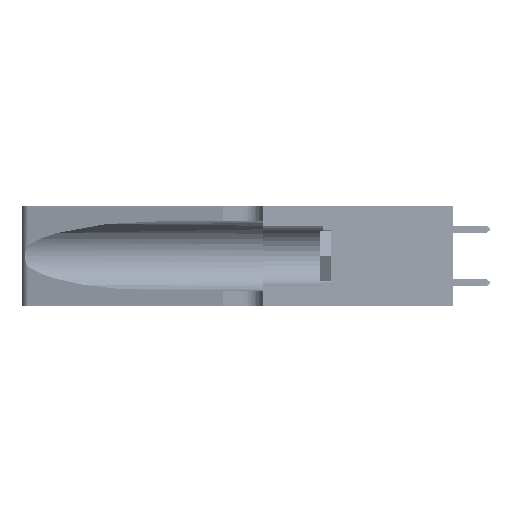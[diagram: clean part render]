
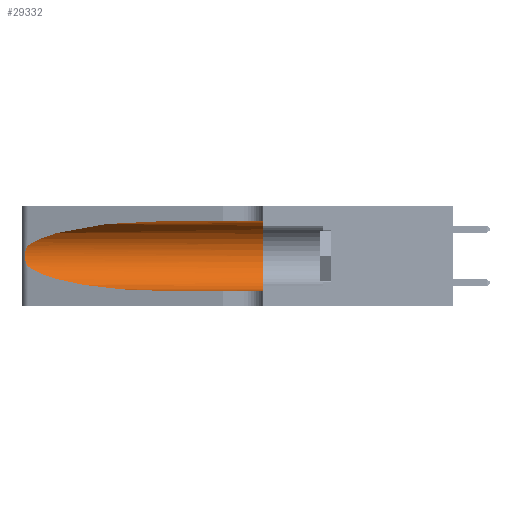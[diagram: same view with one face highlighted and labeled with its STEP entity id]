
A CAD part, left-side view. The second image highlights one B-rep face of the part: STEP entity #29332.
In plain terms, the highlighted cylindrical face has radius 3.308 mm (diameter 6.617 mm), a partial arc.
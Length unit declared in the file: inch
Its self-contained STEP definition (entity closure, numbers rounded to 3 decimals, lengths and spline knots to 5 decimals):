
#169 = CARTESIAN_POINT ( 'NONE',  ( 0.1305, 0.35, 0.31525 ) ) ;
#1890 = VERTEX_POINT ( 'NONE', #169 ) ;
#1937 = CARTESIAN_POINT ( 'NONE',  ( 0.25555, 1.22993, 0.14849 ) ) ;
#3401 = VECTOR ( 'NONE', #18199, 39.37008 ) ;
#4454 = CARTESIAN_POINT ( 'NONE',  ( 0.1305, 0.35, 0.185 ) ) ;
#5947 = CARTESIAN_POINT ( 'NONE',  ( 0.25555, 1.22994, 0.2215 ) ) ;
#6006 = VERTEX_POINT ( 'NONE', #49489 ) ;
#6018 = LINE ( 'NONE', #13987, #3401 ) ;
#6129 = EDGE_CURVE ( 'NONE', #32163, #25042, #22396, .T. ) ;
#7851 =( BOUNDED_CURVE ( )  B_SPLINE_CURVE ( 3, ( #29032, #51303, #33178, #8228 ),
 .UNSPECIFIED., .F., .T. ) 
 B_SPLINE_CURVE_WITH_KNOTS ( ( 4, 4 ),
 ( 1.5708, 2.84003 ),
 .UNSPECIFIED. ) 
 CURVE ( )  GEOMETRIC_REPRESENTATION_ITEM ( )  RATIONAL_B_SPLINE_CURVE ( ( 1., 0.87, 0.87, 1. ) ) 
 REPRESENTATION_ITEM ( '' )  );
#8228 = CARTESIAN_POINT ( 'NONE',  ( 0.25487, 1.22718, 0.22369 ) ) ;
#8542 = LINE ( 'NONE', #27172, #42915 ) ;
#8654 = DIRECTION ( 'NONE',  ( 0., 0., 1. ) ) ;
#10156 = CARTESIAN_POINT ( 'NONE',  ( 0.25787, 1.23484, 0.2124 ) ) ;
#10996 = ORIENTED_EDGE ( 'NONE', *, *, #44188, .F. ) ;
#11939 = CYLINDRICAL_SURFACE ( 'NONE', #45114, 0.13025 ) ;
#12152 = CARTESIAN_POINT ( 'NONE',  ( 0.25487, 1.22718, 0.22369 ) ) ;
#12495 = EDGE_CURVE ( 'NONE', #1890, #6006, #49805, .T. ) ;
#12565 = CARTESIAN_POINT ( 'NONE',  ( 0.1305, 0.72297, 0.31525 ) ) ;
#12991 = CARTESIAN_POINT ( 'NONE',  ( 0.18966, 0.96281, 0.05475 ) ) ;
#13987 = CARTESIAN_POINT ( 'NONE',  ( 0.1305, 1.61858, 0.05475 ) ) ;
#14342 = CARTESIAN_POINT ( 'NONE',  ( 0.26018, 1.23835, 0.19895 ) ) ;
#16954 = VERTEX_POINT ( 'NONE', #12565 ) ;
#17201 = CARTESIAN_POINT ( 'NONE',  ( 0.1305, 0.72297, 0.05475 ) ) ;
#18199 = DIRECTION ( 'NONE',  ( 0., -1., 0. ) ) ;
#18373 = CARTESIAN_POINT ( 'NONE',  ( 0.1305, 1.61858, 0.185 ) ) ;
#18577 = CARTESIAN_POINT ( 'NONE',  ( 0.26075, 1.23896, 0.178 ) ) ;
#22396 =( BOUNDED_CURVE ( )  B_SPLINE_CURVE ( 3, ( #41966, #37869, #12991, #17201 ),
 .UNSPECIFIED., .F., .F. ) 
 B_SPLINE_CURVE_WITH_KNOTS ( ( 4, 4 ),
 ( 3.44316, 4.71239 ),
 .UNSPECIFIED. ) 
 CURVE ( )  GEOMETRIC_REPRESENTATION_ITEM ( )  RATIONAL_B_SPLINE_CURVE ( ( 1., 0.87, 0.87, 1. ) ) 
 REPRESENTATION_ITEM ( '' )  );
#22766 = CARTESIAN_POINT ( 'NONE',  ( 0.25856, 1.23593, 0.16098 ) ) ;
#25042 = VERTEX_POINT ( 'NONE', #27680 ) ;
#25709 = B_SPLINE_CURVE_WITH_KNOTS ( 'NONE', 3,
 ( #30959, #5947, #35097, #10156, #39177, #14342, #43284, #18577, #47398, #22766, #51499, #26936, #1937, #31132 ),
 .UNSPECIFIED., .F., .F.,
 ( 4, 2, 2, 2, 2, 2, 4 ),
 ( 0., 0.00027, 0.00053, 0.00107, 0.0016, 0.00187, 0.00214 ),
 .UNSPECIFIED. ) ;
#26936 = CARTESIAN_POINT ( 'NONE',  ( 0.25639, 1.23186, 0.15144 ) ) ;
#27172 = CARTESIAN_POINT ( 'NONE',  ( 0.1305, 1.61858, 0.31525 ) ) ;
#27680 = CARTESIAN_POINT ( 'NONE',  ( 0.1305, 0.72297, 0.05475 ) ) ;
#29032 = CARTESIAN_POINT ( 'NONE',  ( 0.1305, 0.72297, 0.31525 ) ) ;
#29332 = ADVANCED_FACE ( 'NONE', ( #44983 ), #11939, .F. ) ;
#30952 = DIRECTION ( 'NONE',  ( 0., -1., 0. ) ) ;
#30959 = CARTESIAN_POINT ( 'NONE',  ( 0.25487, 1.22718, 0.22369 ) ) ;
#31132 = CARTESIAN_POINT ( 'NONE',  ( 0.25487, 1.22718, 0.14631 ) ) ;
#31355 = DIRECTION ( 'NONE',  ( 0., -1., 0. ) ) ;
#31942 = CARTESIAN_POINT ( 'NONE',  ( 0.25487, 1.22718, 0.14631 ) ) ;
#32163 = VERTEX_POINT ( 'NONE', #31942 ) ;
#33135 = AXIS2_PLACEMENT_3D ( 'NONE', #4454, #33610, #8654 ) ;
#33178 = CARTESIAN_POINT ( 'NONE',  ( 0.2373, 1.15595, 0.28018 ) ) ;
#33610 = DIRECTION ( 'NONE',  ( 0., 1., 0. ) ) ;
#35097 = CARTESIAN_POINT ( 'NONE',  ( 0.25639, 1.23184, 0.21858 ) ) ;
#35656 = ORIENTED_EDGE ( 'NONE', *, *, #6129, .T. ) ;
#36165 = EDGE_CURVE ( 'NONE', #16954, #40927, #7851, .T. ) ;
#37869 = CARTESIAN_POINT ( 'NONE',  ( 0.2373, 1.15595, 0.08982 ) ) ;
#39177 = CARTESIAN_POINT ( 'NONE',  ( 0.25854, 1.2359, 0.20912 ) ) ;
#39926 = ORIENTED_EDGE ( 'NONE', *, *, #47368, .T. ) ;
#40927 = VERTEX_POINT ( 'NONE', #12152 ) ;
#41966 = CARTESIAN_POINT ( 'NONE',  ( 0.25487, 1.22718, 0.14631 ) ) ;
#42675 = EDGE_CURVE ( 'NONE', #25042, #6006, #6018, .T. ) ;
#42915 = VECTOR ( 'NONE', #31355, 39.37008 ) ;
#43284 = CARTESIAN_POINT ( 'NONE',  ( 0.26075, 1.23896, 0.19203 ) ) ;
#43776 = ORIENTED_EDGE ( 'NONE', *, *, #42675, .T. ) ;
#44188 = EDGE_CURVE ( 'NONE', #16954, #1890, #8542, .T. ) ;
#44983 = FACE_OUTER_BOUND ( 'NONE', #50782, .T. ) ;
#45114 = AXIS2_PLACEMENT_3D ( 'NONE', #18373, #30952, #47023 ) ;
#47023 = DIRECTION ( 'NONE',  ( 0., 0., -1. ) ) ;
#47368 = EDGE_CURVE ( 'NONE', #40927, #32163, #25709, .T. ) ;
#47398 = CARTESIAN_POINT ( 'NONE',  ( 0.26017, 1.23833, 0.17102 ) ) ;
#47873 = ORIENTED_EDGE ( 'NONE', *, *, #36165, .T. ) ;
#49489 = CARTESIAN_POINT ( 'NONE',  ( 0.1305, 0.35, 0.05475 ) ) ;
#49805 = CIRCLE ( 'NONE', #33135, 0.13025 ) ;
#50782 = EDGE_LOOP ( 'NONE', ( #47873, #39926, #35656, #43776, #53191, #10996 ) ) ;
#51303 = CARTESIAN_POINT ( 'NONE',  ( 0.18966, 0.96281, 0.31525 ) ) ;
#51499 = CARTESIAN_POINT ( 'NONE',  ( 0.25789, 1.23486, 0.15765 ) ) ;
#53191 = ORIENTED_EDGE ( 'NONE', *, *, #12495, .F. ) ;
